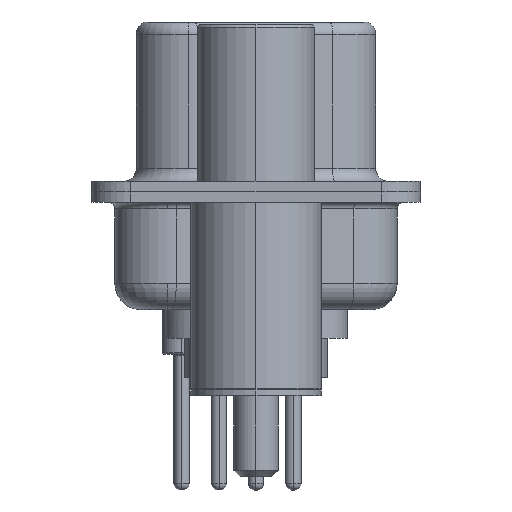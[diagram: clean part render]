
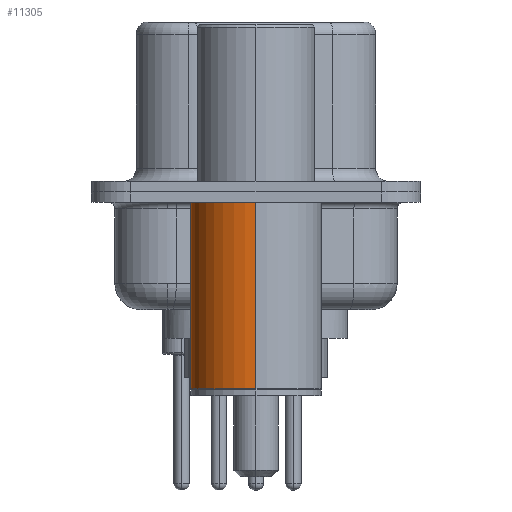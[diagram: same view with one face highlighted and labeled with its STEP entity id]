
A CAD part, left-side view. The second image highlights one B-rep face of the part: STEP entity #11305.
In plain terms, the highlighted cylindrical face has radius 2.5 mm (diameter 5 mm), a partial arc.
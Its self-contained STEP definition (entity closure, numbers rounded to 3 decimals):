
#253 = DIRECTION ( 'NONE',  ( 0., 0., 1. ) ) ;
#344 = VERTEX_POINT ( 'NONE', #23505 ) ;
#444 = DIRECTION ( 'NONE',  ( 1., 0., 0. ) ) ;
#2429 = EDGE_LOOP ( 'NONE', ( #14586, #8649, #18875, #7383 ) ) ;
#5923 = CIRCLE ( 'NONE', #20957, 2.5 ) ;
#7060 = LINE ( 'NONE', #14548, #12073 ) ;
#7140 = DIRECTION ( 'NONE',  ( 1., 0., 0. ) ) ;
#7383 = ORIENTED_EDGE ( 'NONE', *, *, #24208, .F. ) ;
#7448 = LINE ( 'NONE', #9088, #11807 ) ;
#7822 = FACE_OUTER_BOUND ( 'NONE', #2429, .T. ) ;
#8014 = EDGE_CURVE ( 'NONE', #11862, #344, #5923, .T. ) ;
#8457 = CIRCLE ( 'NONE', #25337, 2.5 ) ;
#8649 = ORIENTED_EDGE ( 'NONE', *, *, #13229, .T. ) ;
#8870 = DIRECTION ( 'NONE',  ( 0., 0., 1. ) ) ;
#9088 = CARTESIAN_POINT ( 'NONE',  ( 2.5, 0., 0.581 ) ) ;
#10745 = CARTESIAN_POINT ( 'NONE',  ( 0., 0., 0.581 ) ) ;
#11094 = VERTEX_POINT ( 'NONE', #22998 ) ;
#11255 = DIRECTION ( 'NONE',  ( 0., 0., 1. ) ) ;
#11305 = ADVANCED_FACE ( 'NONE', ( #7822 ), #20786, .T. ) ;
#11479 = VERTEX_POINT ( 'NONE', #17179 ) ;
#11795 = EDGE_CURVE ( 'NONE', #11479, #11094, #8457, .T. ) ;
#11807 = VECTOR ( 'NONE', #24011, 1000. ) ;
#11862 = VERTEX_POINT ( 'NONE', #17483 ) ;
#12073 = VECTOR ( 'NONE', #12689, 1000. ) ;
#12689 = DIRECTION ( 'NONE',  ( 0., 0., 1. ) ) ;
#13229 = EDGE_CURVE ( 'NONE', #344, #11094, #7060, .T. ) ;
#14548 = CARTESIAN_POINT ( 'NONE',  ( -2.5, 0., 0.581 ) ) ;
#14586 = ORIENTED_EDGE ( 'NONE', *, *, #8014, .T. ) ;
#17179 = CARTESIAN_POINT ( 'NONE',  ( 2.5, 0., -0.4 ) ) ;
#17483 = CARTESIAN_POINT ( 'NONE',  ( 2.5, 0., -7.525 ) ) ;
#18875 = ORIENTED_EDGE ( 'NONE', *, *, #11795, .F. ) ;
#20786 = CYLINDRICAL_SURFACE ( 'NONE', #25495, 2.5 ) ;
#20957 = AXIS2_PLACEMENT_3D ( 'NONE', #22139, #11255, #7140 ) ;
#22139 = CARTESIAN_POINT ( 'NONE',  ( 0., 0., -7.525 ) ) ;
#22998 = CARTESIAN_POINT ( 'NONE',  ( -2.5, 0., -0.4 ) ) ;
#23505 = CARTESIAN_POINT ( 'NONE',  ( -2.5, 0., -7.525 ) ) ;
#24011 = DIRECTION ( 'NONE',  ( 0., 0., 1. ) ) ;
#24208 = EDGE_CURVE ( 'NONE', #11862, #11479, #7448, .T. ) ;
#25337 = AXIS2_PLACEMENT_3D ( 'NONE', #26318, #8870, #444 ) ;
#25495 = AXIS2_PLACEMENT_3D ( 'NONE', #10745, #253, #26028 ) ;
#26028 = DIRECTION ( 'NONE',  ( 1., 0., 0. ) ) ;
#26318 = CARTESIAN_POINT ( 'NONE',  ( 0., 0., -0.4 ) ) ;
